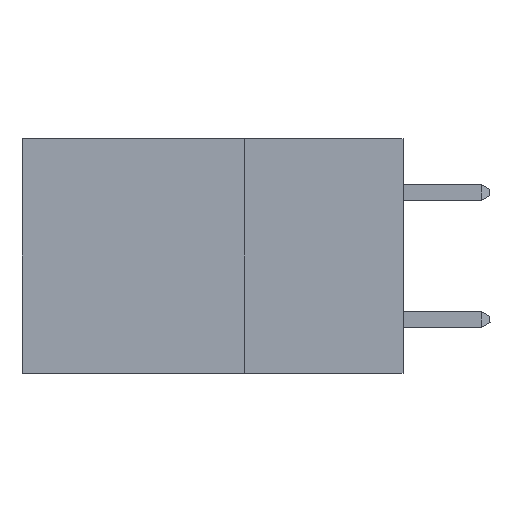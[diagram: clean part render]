
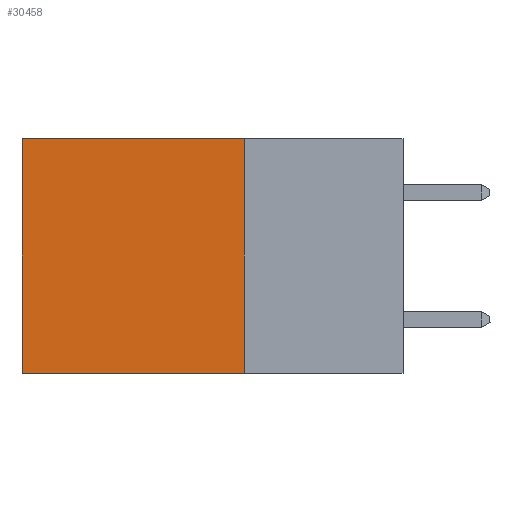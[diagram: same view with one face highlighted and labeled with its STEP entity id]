
A CAD part, left-side view. The second image highlights one B-rep face of the part: STEP entity #30458.
In plain terms, the highlighted planar face has unit normal (-1, 0, 0).
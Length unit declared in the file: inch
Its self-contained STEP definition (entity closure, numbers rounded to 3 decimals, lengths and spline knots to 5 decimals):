
#1140 = LINE ( 'NONE', #5331, #22578 ) ;
#1288 = DIRECTION ( 'NONE',  ( 0., 1., 0. ) ) ;
#1321 = EDGE_CURVE ( 'NONE', #32506, #14164, #13308, .T. ) ;
#1594 = CARTESIAN_POINT ( 'NONE',  ( 0.2875, 0.25, 0. ) ) ;
#3603 = VERTEX_POINT ( 'NONE', #18974 ) ;
#4173 = DIRECTION ( 'NONE',  ( 0., 0., -1. ) ) ;
#4607 = ORIENTED_EDGE ( 'NONE', *, *, #1321, .F. ) ;
#5331 = CARTESIAN_POINT ( 'NONE',  ( 0.2875, 0.6, 0. ) ) ;
#5886 = DIRECTION ( 'NONE',  ( 0., 0., -1. ) ) ;
#8143 = DIRECTION ( 'NONE',  ( 0., 0., -1. ) ) ;
#10008 = EDGE_CURVE ( 'NONE', #23051, #3603, #1140, .T. ) ;
#11544 = CARTESIAN_POINT ( 'NONE',  ( 0.2875, 0.25, 0. ) ) ;
#13308 = LINE ( 'NONE', #19310, #25515 ) ;
#14062 = VECTOR ( 'NONE', #1288, 39.37008 ) ;
#14164 = VERTEX_POINT ( 'NONE', #25573 ) ;
#15918 = EDGE_CURVE ( 'NONE', #32506, #23051, #24655, .T. ) ;
#17754 = ORIENTED_EDGE ( 'NONE', *, *, #23295, .F. ) ;
#18974 = CARTESIAN_POINT ( 'NONE',  ( 0.2875, 0.6, -0.37 ) ) ;
#19310 = CARTESIAN_POINT ( 'NONE',  ( 0.2875, 0.25, 0. ) ) ;
#19350 = AXIS2_PLACEMENT_3D ( 'NONE', #1594, #30207, #4173 ) ;
#19353 = LINE ( 'NONE', #27434, #30347 ) ;
#20104 = PLANE ( 'NONE',  #19350 ) ;
#22578 = VECTOR ( 'NONE', #8143, 39.37008 ) ;
#23051 = VERTEX_POINT ( 'NONE', #25981 ) ;
#23295 = EDGE_CURVE ( 'NONE', #14164, #3603, #19353, .T. ) ;
#24232 = FACE_OUTER_BOUND ( 'NONE', #26491, .T. ) ;
#24655 = LINE ( 'NONE', #11544, #14062 ) ;
#25515 = VECTOR ( 'NONE', #5886, 39.37008 ) ;
#25573 = CARTESIAN_POINT ( 'NONE',  ( 0.2875, 0.25, -0.37 ) ) ;
#25981 = CARTESIAN_POINT ( 'NONE',  ( 0.2875, 0.6, 0. ) ) ;
#26491 = EDGE_LOOP ( 'NONE', ( #32967, #17754, #4607, #33309 ) ) ;
#27434 = CARTESIAN_POINT ( 'NONE',  ( 0.2875, 0.25, -0.37 ) ) ;
#27795 = CARTESIAN_POINT ( 'NONE',  ( 0.2875, 0.25, 0. ) ) ;
#30207 = DIRECTION ( 'NONE',  ( 1., 0., 0. ) ) ;
#30347 = VECTOR ( 'NONE', #32158, 39.37008 ) ;
#30458 = ADVANCED_FACE ( 'NONE', ( #24232 ), #20104, .F. ) ;
#32158 = DIRECTION ( 'NONE',  ( 0., 1., 0. ) ) ;
#32506 = VERTEX_POINT ( 'NONE', #27795 ) ;
#32967 = ORIENTED_EDGE ( 'NONE', *, *, #10008, .T. ) ;
#33309 = ORIENTED_EDGE ( 'NONE', *, *, #15918, .T. ) ;
